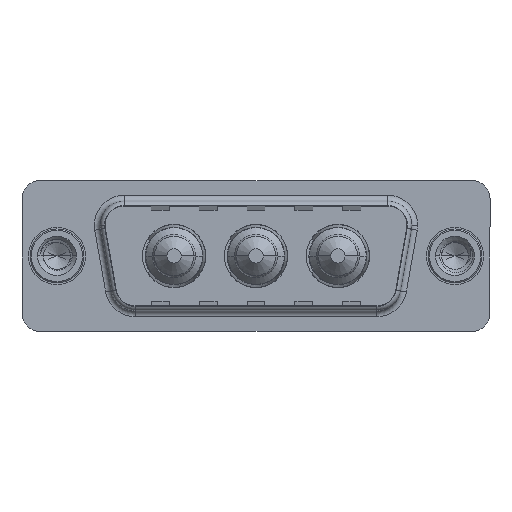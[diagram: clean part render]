
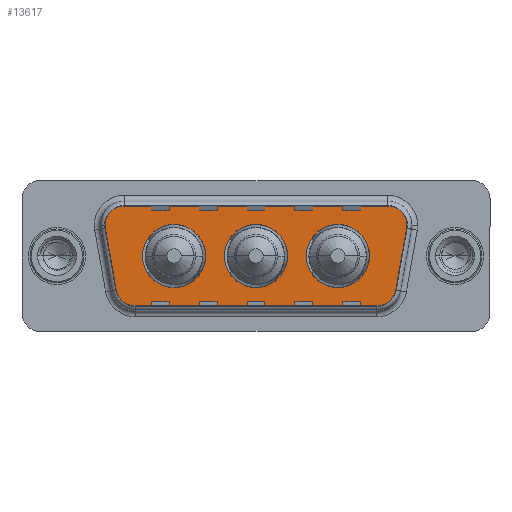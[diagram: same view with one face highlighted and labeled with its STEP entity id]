
A CAD part, top view. The second image highlights one B-rep face of the part: STEP entity #13617.
In plain terms, the highlighted planar face has unit normal (0, 0, 1).
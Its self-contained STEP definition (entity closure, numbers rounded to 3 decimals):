
#368 = CIRCLE ( 'NONE', #4522, 2.65 ) ;
#453 = PLANE ( 'NONE',  #8941 ) ;
#455 = CARTESIAN_POINT ( 'NONE',  ( 9.8, 0., 0. ) ) ;
#462 = CARTESIAN_POINT ( 'NONE',  ( 5.411, 4.9, 0. ) ) ;
#509 = EDGE_LOOP ( 'NONE', ( #1603, #1299 ) ) ;
#519 = DIRECTION ( 'NONE',  ( 0., 0., 1. ) ) ;
#589 = CARTESIAN_POINT ( 'NONE',  ( 19.3, 0., 0. ) ) ;
#714 = ORIENTED_EDGE ( 'NONE', *, *, #4204, .T. ) ;
#717 = EDGE_LOOP ( 'NONE', ( #5523, #3065, #714, #1769, #17704, #5793, #5552, #16056, #11918 ) ) ;
#775 = VECTOR ( 'NONE', #6622, 1000. ) ;
#872 = DIRECTION ( 'NONE',  ( 1., 0., 0. ) ) ;
#941 = VERTEX_POINT ( 'NONE', #589 ) ;
#1001 = EDGE_CURVE ( 'NONE', #13983, #19190, #10944, .T. ) ;
#1021 = CARTESIAN_POINT ( 'NONE',  ( 7.15, 0., 0. ) ) ;
#1133 = DIRECTION ( 'NONE',  ( 0., 0., 1. ) ) ;
#1299 = ORIENTED_EDGE ( 'NONE', *, *, #15341, .F. ) ;
#1344 = FACE_OUTER_BOUND ( 'NONE', #717, .T. ) ;
#1593 = EDGE_CURVE ( 'NONE', #3884, #18789, #19586, .T. ) ;
#1603 = ORIENTED_EDGE ( 'NONE', *, *, #1614, .F. ) ;
#1614 = EDGE_CURVE ( 'NONE', #941, #19768, #5330, .T. ) ;
#1683 = AXIS2_PLACEMENT_3D ( 'NONE', #11857, #2606, #13397 ) ;
#1769 = ORIENTED_EDGE ( 'NONE', *, *, #10079, .T. ) ;
#1962 = DIRECTION ( 'NONE',  ( 1., 0., 0. ) ) ;
#2310 = VERTEX_POINT ( 'NONE', #19647 ) ;
#2413 = EDGE_CURVE ( 'NONE', #7888, #9571, #12101, .T. ) ;
#2606 = DIRECTION ( 'NONE',  ( 0., 0., 1. ) ) ;
#2968 = EDGE_CURVE ( 'NONE', #16957, #7888, #12556, .T. ) ;
#2977 = CARTESIAN_POINT ( 'NONE',  ( 6.434, -4.9, 0. ) ) ;
#3065 = ORIENTED_EDGE ( 'NONE', *, *, #1593, .T. ) ;
#3388 = DIRECTION ( 'NONE',  ( -1., 0., 0. ) ) ;
#3506 = DIRECTION ( 'NONE',  ( 1., 0., 0. ) ) ;
#3884 = VERTEX_POINT ( 'NONE', #7679 ) ;
#3948 = ORIENTED_EDGE ( 'NONE', *, *, #14234, .F. ) ;
#4202 = AXIS2_PLACEMENT_3D ( 'NONE', #4240, #15057, #5811 ) ;
#4204 = EDGE_CURVE ( 'NONE', #18789, #4332, #13493, .T. ) ;
#4240 = CARTESIAN_POINT ( 'NONE',  ( 27.889, 2.9, 0. ) ) ;
#4332 = VERTEX_POINT ( 'NONE', #15478 ) ;
#4416 = CIRCLE ( 'NONE', #12957, 2. ) ;
#4522 = AXIS2_PLACEMENT_3D ( 'NONE', #455, #11216, #1962 ) ;
#5313 = CARTESIAN_POINT ( 'NONE',  ( 6.434, -2.9, 0. ) ) ;
#5330 = CIRCLE ( 'NONE', #14466, 2.65 ) ;
#5384 = FACE_BOUND ( 'NONE', #7455, .T. ) ;
#5523 = ORIENTED_EDGE ( 'NONE', *, *, #14638, .T. ) ;
#5552 = ORIENTED_EDGE ( 'NONE', *, *, #2968, .T. ) ;
#5793 = ORIENTED_EDGE ( 'NONE', *, *, #17542, .T. ) ;
#5811 = DIRECTION ( 'NONE',  ( -1., 0., 0. ) ) ;
#5824 = VECTOR ( 'NONE', #9085, 1000. ) ;
#5978 = DIRECTION ( 'NONE',  ( -1., 0., 0. ) ) ;
#6535 = CARTESIAN_POINT ( 'NONE',  ( 26.866, -2.9, 0. ) ) ;
#6622 = DIRECTION ( 'NONE',  ( 0.174, -0.985, 0. ) ) ;
#6627 = AXIS2_PLACEMENT_3D ( 'NONE', #17412, #8183, #18966 ) ;
#6819 = EDGE_CURVE ( 'NONE', #10371, #8076, #11202, .T. ) ;
#6964 = CARTESIAN_POINT ( 'NONE',  ( 3.441, 2.553, 0. ) ) ;
#7076 = VECTOR ( 'NONE', #3388, 1000. ) ;
#7182 = ORIENTED_EDGE ( 'NONE', *, *, #11264, .F. ) ;
#7285 = CARTESIAN_POINT ( 'NONE',  ( 5.411, 2.9, 0. ) ) ;
#7289 = DIRECTION ( 'NONE',  ( 0., 0., 1. ) ) ;
#7455 = EDGE_LOOP ( 'NONE', ( #8348, #3948 ) ) ;
#7536 = DIRECTION ( 'NONE',  ( 0., 0., 1. ) ) ;
#7545 = EDGE_CURVE ( 'NONE', #9571, #2310, #16955, .T. ) ;
#7564 = CIRCLE ( 'NONE', #6627, 2.65 ) ;
#7679 = CARTESIAN_POINT ( 'NONE',  ( 28.836, -3.247, 0. ) ) ;
#7888 = VERTEX_POINT ( 'NONE', #8628 ) ;
#8076 = VERTEX_POINT ( 'NONE', #13609 ) ;
#8183 = DIRECTION ( 'NONE',  ( 0., 0., 1. ) ) ;
#8348 = ORIENTED_EDGE ( 'NONE', *, *, #15309, .F. ) ;
#8571 = CARTESIAN_POINT ( 'NONE',  ( 3.441, 2.553, 0. ) ) ;
#8628 = CARTESIAN_POINT ( 'NONE',  ( 4.464, -3.247, 0. ) ) ;
#8836 = DIRECTION ( 'NONE',  ( 1., 0., 0. ) ) ;
#8941 = AXIS2_PLACEMENT_3D ( 'NONE', #6535, #12750, #3506 ) ;
#9085 = DIRECTION ( 'NONE',  ( 0.174, 0.985, 0. ) ) ;
#9242 = CARTESIAN_POINT ( 'NONE',  ( 29.859, 2.553, 0. ) ) ;
#9571 = VERTEX_POINT ( 'NONE', #14003 ) ;
#9724 = CARTESIAN_POINT ( 'NONE',  ( 26.866, -2.9, 0. ) ) ;
#9799 = CARTESIAN_POINT ( 'NONE',  ( 26.15, 0., 0. ) ) ;
#9864 = CIRCLE ( 'NONE', #1683, 2.65 ) ;
#10079 = EDGE_CURVE ( 'NONE', #4332, #10371, #19287, .T. ) ;
#10325 = CARTESIAN_POINT ( 'NONE',  ( 9.8, 0., 0. ) ) ;
#10371 = VERTEX_POINT ( 'NONE', #18845 ) ;
#10944 = CIRCLE ( 'NONE', #11099, 2.65 ) ;
#11099 = AXIS2_PLACEMENT_3D ( 'NONE', #17896, #14272, #872 ) ;
#11188 = EDGE_LOOP ( 'NONE', ( #11248, #7182 ) ) ;
#11202 = LINE ( 'NONE', #462, #7076 ) ;
#11216 = DIRECTION ( 'NONE',  ( 0., 0., 1. ) ) ;
#11248 = ORIENTED_EDGE ( 'NONE', *, *, #1001, .F. ) ;
#11254 = AXIS2_PLACEMENT_3D ( 'NONE', #5313, #7289, #5978 ) ;
#11264 = EDGE_CURVE ( 'NONE', #19190, #13983, #9864, .T. ) ;
#11285 = DIRECTION ( 'NONE',  ( 1., 0., 0. ) ) ;
#11857 = CARTESIAN_POINT ( 'NONE',  ( 23.5, 0., 0. ) ) ;
#11898 = DIRECTION ( 'NONE',  ( 1., 0., 0. ) ) ;
#11918 = ORIENTED_EDGE ( 'NONE', *, *, #7545, .T. ) ;
#12101 = CIRCLE ( 'NONE', #11254, 2. ) ;
#12303 = AXIS2_PLACEMENT_3D ( 'NONE', #10325, #1133, #11898 ) ;
#12556 = LINE ( 'NONE', #6964, #775 ) ;
#12685 = AXIS2_PLACEMENT_3D ( 'NONE', #16778, #7536, #18339 ) ;
#12750 = DIRECTION ( 'NONE',  ( 0., 0., 1. ) ) ;
#12857 = VECTOR ( 'NONE', #13768, 1000. ) ;
#12957 = AXIS2_PLACEMENT_3D ( 'NONE', #9724, #519, #11285 ) ;
#13130 = FACE_BOUND ( 'NONE', #11188, .T. ) ;
#13236 = AXIS2_PLACEMENT_3D ( 'NONE', #7285, #18093, #8836 ) ;
#13397 = DIRECTION ( 'NONE',  ( 1., 0., 0. ) ) ;
#13493 = CIRCLE ( 'NONE', #12685, 2. ) ;
#13609 = CARTESIAN_POINT ( 'NONE',  ( 5.411, 4.9, 0. ) ) ;
#13617 = ADVANCED_FACE ( 'NONE', ( #17235, #13130, #5384, #1344 ), #453, .T. ) ;
#13768 = DIRECTION ( 'NONE',  ( 1., 0., 0. ) ) ;
#13864 = CIRCLE ( 'NONE', #12303, 2.65 ) ;
#13968 = VERTEX_POINT ( 'NONE', #14400 ) ;
#13983 = VERTEX_POINT ( 'NONE', #9799 ) ;
#14003 = CARTESIAN_POINT ( 'NONE',  ( 6.434, -4.9, 0. ) ) ;
#14234 = EDGE_CURVE ( 'NONE', #15502, #13968, #13864, .T. ) ;
#14272 = DIRECTION ( 'NONE',  ( 0., 0., 1. ) ) ;
#14400 = CARTESIAN_POINT ( 'NONE',  ( 12.45, 0., 0. ) ) ;
#14466 = AXIS2_PLACEMENT_3D ( 'NONE', #18607, #18568, #17671 ) ;
#14638 = EDGE_CURVE ( 'NONE', #2310, #3884, #4416, .T. ) ;
#14964 = CIRCLE ( 'NONE', #13236, 2. ) ;
#14999 = CARTESIAN_POINT ( 'NONE',  ( 14., 0., 0. ) ) ;
#15057 = DIRECTION ( 'NONE',  ( 0., 0., 1. ) ) ;
#15296 = CARTESIAN_POINT ( 'NONE',  ( 20.85, 0., 0. ) ) ;
#15309 = EDGE_CURVE ( 'NONE', #13968, #15502, #368, .T. ) ;
#15341 = EDGE_CURVE ( 'NONE', #19768, #941, #7564, .T. ) ;
#15478 = CARTESIAN_POINT ( 'NONE',  ( 29.889, 2.9, 0. ) ) ;
#15502 = VERTEX_POINT ( 'NONE', #1021 ) ;
#15976 = CARTESIAN_POINT ( 'NONE',  ( 29.859, 2.553, 0. ) ) ;
#16056 = ORIENTED_EDGE ( 'NONE', *, *, #2413, .T. ) ;
#16778 = CARTESIAN_POINT ( 'NONE',  ( 27.889, 2.9, 0. ) ) ;
#16955 = LINE ( 'NONE', #2977, #12857 ) ;
#16957 = VERTEX_POINT ( 'NONE', #8571 ) ;
#17235 = FACE_BOUND ( 'NONE', #509, .T. ) ;
#17412 = CARTESIAN_POINT ( 'NONE',  ( 16.65, 0., 0. ) ) ;
#17542 = EDGE_CURVE ( 'NONE', #8076, #16957, #14964, .T. ) ;
#17671 = DIRECTION ( 'NONE',  ( 1., 0., 0. ) ) ;
#17704 = ORIENTED_EDGE ( 'NONE', *, *, #6819, .T. ) ;
#17896 = CARTESIAN_POINT ( 'NONE',  ( 23.5, 0., 0. ) ) ;
#18093 = DIRECTION ( 'NONE',  ( 0., 0., 1. ) ) ;
#18339 = DIRECTION ( 'NONE',  ( -1., 0., 0. ) ) ;
#18568 = DIRECTION ( 'NONE',  ( 0., 0., 1. ) ) ;
#18607 = CARTESIAN_POINT ( 'NONE',  ( 16.65, 0., 0. ) ) ;
#18789 = VERTEX_POINT ( 'NONE', #15976 ) ;
#18845 = CARTESIAN_POINT ( 'NONE',  ( 27.889, 4.9, 0. ) ) ;
#18966 = DIRECTION ( 'NONE',  ( 1., 0., 0. ) ) ;
#19190 = VERTEX_POINT ( 'NONE', #15296 ) ;
#19287 = CIRCLE ( 'NONE', #4202, 2. ) ;
#19586 = LINE ( 'NONE', #9242, #5824 ) ;
#19647 = CARTESIAN_POINT ( 'NONE',  ( 26.866, -4.9, 0. ) ) ;
#19768 = VERTEX_POINT ( 'NONE', #14999 ) ;
